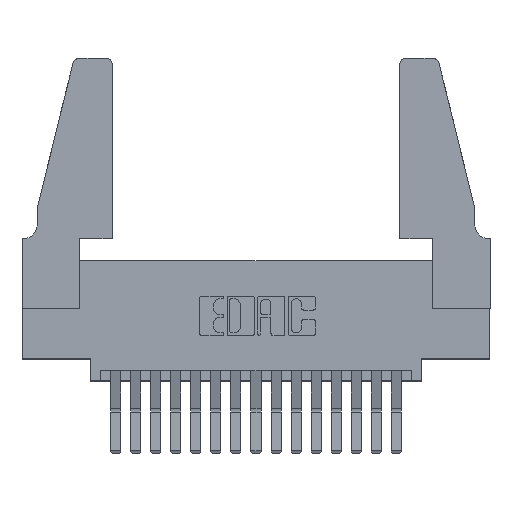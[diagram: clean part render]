
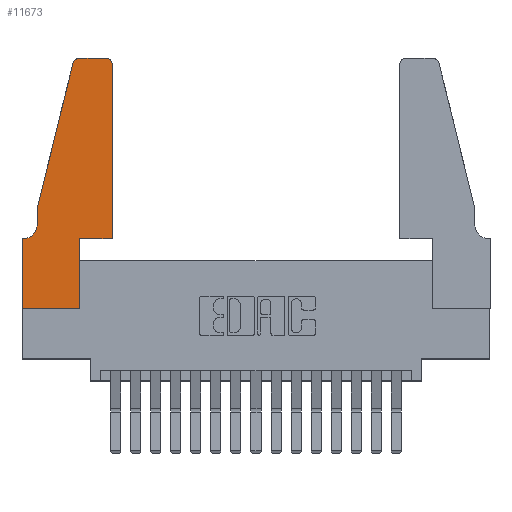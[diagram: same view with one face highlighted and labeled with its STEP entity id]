
A CAD part, top view. The second image highlights one B-rep face of the part: STEP entity #11673.
In plain terms, the highlighted planar face has unit normal (0, 0, 1).
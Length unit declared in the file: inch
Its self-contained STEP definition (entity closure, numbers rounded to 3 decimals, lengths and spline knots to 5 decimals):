
#372 = PLANE ( 'NONE',  #6034 ) ;
#391 = CARTESIAN_POINT ( 'NONE',  ( 0.2605, 1.25, 0.37 ) ) ;
#405 = VECTOR ( 'NONE', #438, 39.37008 ) ;
#438 = DIRECTION ( 'NONE',  ( 0., -1., 0. ) ) ;
#441 = CARTESIAN_POINT ( 'NONE',  ( 0.0755, 0.35, 0.37 ) ) ;
#473 = EDGE_CURVE ( 'NONE', #3197, #6181, #17310, .T. ) ;
#715 = CARTESIAN_POINT ( 'NONE',  ( 0., 0., 0.37 ) ) ;
#916 = VECTOR ( 'NONE', #14124, 39.37008 ) ;
#1012 = VECTOR ( 'NONE', #6200, 39.37008 ) ;
#1357 = DIRECTION ( 'NONE',  ( 1., 0., 0. ) ) ;
#1380 = CARTESIAN_POINT ( 'NONE',  ( 0., 0., 0.37 ) ) ;
#1688 = CARTESIAN_POINT ( 'NONE',  ( 0.4205, 1.25, 0.37 ) ) ;
#1715 = DIRECTION ( 'NONE',  ( 0., 0., 1. ) ) ;
#1775 = CARTESIAN_POINT ( 'NONE',  ( 0.4505, 0.35, 0.37 ) ) ;
#2473 = AXIS2_PLACEMENT_3D ( 'NONE', #11546, #9897, #15420 ) ;
#2487 = ORIENTED_EDGE ( 'NONE', *, *, #16562, .T. ) ;
#2564 = EDGE_CURVE ( 'NONE', #14074, #11543, #9876, .T. ) ;
#2922 = LINE ( 'NONE', #5318, #5719 ) ;
#3162 = DIRECTION ( 'NONE',  ( 0., 0., 1. ) ) ;
#3197 = VERTEX_POINT ( 'NONE', #17264 ) ;
#3398 = EDGE_CURVE ( 'NONE', #13388, #10427, #12030, .T. ) ;
#3519 = DIRECTION ( 'NONE',  ( 0., 1., 0. ) ) ;
#3649 = VERTEX_POINT ( 'NONE', #1775 ) ;
#4093 = ORIENTED_EDGE ( 'NONE', *, *, #11436, .T. ) ;
#4579 = DIRECTION ( 'NONE',  ( 0., 0., -1. ) ) ;
#4583 = CARTESIAN_POINT ( 'NONE',  ( 0.2865, 0., 0.37 ) ) ;
#4635 = VECTOR ( 'NONE', #5634, 39.37008 ) ;
#5318 = CARTESIAN_POINT ( 'NONE',  ( 0.4505, 0.35, 0.37 ) ) ;
#5634 = DIRECTION ( 'NONE',  ( -1., 0., 0. ) ) ;
#5673 = VERTEX_POINT ( 'NONE', #15279 ) ;
#5719 = VECTOR ( 'NONE', #12134, 39.37008 ) ;
#5816 = DIRECTION ( 'NONE',  ( 1., 0., 0. ) ) ;
#6004 = ORIENTED_EDGE ( 'NONE', *, *, #15431, .T. ) ;
#6034 = AXIS2_PLACEMENT_3D ( 'NONE', #14144, #3162, #8684 ) ;
#6181 = VERTEX_POINT ( 'NONE', #12402 ) ;
#6200 = DIRECTION ( 'NONE',  ( 1., 0., 0. ) ) ;
#6278 = CIRCLE ( 'NONE', #2473, 0.03 ) ;
#6533 = LINE ( 'NONE', #11529, #17296 ) ;
#6544 = FACE_OUTER_BOUND ( 'NONE', #16868, .T. ) ;
#6876 = CARTESIAN_POINT ( 'NONE',  ( 0.0755, 0.5, 0.37 ) ) ;
#7220 = DIRECTION ( 'NONE',  ( -1., 0., 0. ) ) ;
#8450 = ORIENTED_EDGE ( 'NONE', *, *, #473, .T. ) ;
#8670 = LINE ( 'NONE', #11311, #916 ) ;
#8684 = DIRECTION ( 'NONE',  ( 1., 0., 0. ) ) ;
#9327 = ORIENTED_EDGE ( 'NONE', *, *, #9500, .T. ) ;
#9500 = EDGE_CURVE ( 'NONE', #10845, #11806, #11365, .T. ) ;
#9577 = LINE ( 'NONE', #391, #4635 ) ;
#9876 = LINE ( 'NONE', #15399, #405 ) ;
#9897 = DIRECTION ( 'NONE',  ( 0., 0., 1. ) ) ;
#10202 = EDGE_CURVE ( 'NONE', #3649, #5673, #2922, .T. ) ;
#10216 = LINE ( 'NONE', #6876, #16232 ) ;
#10281 = ORIENTED_EDGE ( 'NONE', *, *, #10202, .T. ) ;
#10427 = VERTEX_POINT ( 'NONE', #4583 ) ;
#10845 = VERTEX_POINT ( 'NONE', #13632 ) ;
#10885 = EDGE_CURVE ( 'NONE', #12292, #3649, #16460, .T. ) ;
#11030 = DIRECTION ( 'NONE',  ( -0.239, -0.971, 0. ) ) ;
#11064 = AXIS2_PLACEMENT_3D ( 'NONE', #14232, #1715, #5816 ) ;
#11311 = CARTESIAN_POINT ( 'NONE',  ( 0., 0., 0.37 ) ) ;
#11365 = CIRCLE ( 'NONE', #11064, 0.03 ) ;
#11436 = EDGE_CURVE ( 'NONE', #11806, #14074, #10216, .T. ) ;
#11529 = CARTESIAN_POINT ( 'NONE',  ( 0.2865, 0.35, 0.37 ) ) ;
#11543 = VERTEX_POINT ( 'NONE', #13845 ) ;
#11546 = CARTESIAN_POINT ( 'NONE',  ( 0.4205, 1.22, 0.37 ) ) ;
#11548 = VERTEX_POINT ( 'NONE', #1688 ) ;
#11673 = ADVANCED_FACE ( 'NONE', ( #6544 ), #372, .T. ) ;
#11806 = VERTEX_POINT ( 'NONE', #11903 ) ;
#11883 = ORIENTED_EDGE ( 'NONE', *, *, #10885, .T. ) ;
#11903 = CARTESIAN_POINT ( 'NONE',  ( 0.25487, 1.22718, 0.37 ) ) ;
#12030 = LINE ( 'NONE', #715, #1012 ) ;
#12134 = DIRECTION ( 'NONE',  ( 0., 1., 0. ) ) ;
#12172 = ORIENTED_EDGE ( 'NONE', *, *, #17451, .T. ) ;
#12280 = CARTESIAN_POINT ( 'NONE',  ( 0.0755, 0.5, 0.37 ) ) ;
#12287 = EDGE_CURVE ( 'NONE', #6181, #13388, #8670, .T. ) ;
#12292 = VERTEX_POINT ( 'NONE', #16890 ) ;
#12402 = CARTESIAN_POINT ( 'NONE',  ( 0., 0.35, 0.37 ) ) ;
#12424 = AXIS2_PLACEMENT_3D ( 'NONE', #15568, #4579, #14301 ) ;
#12638 = CIRCLE ( 'NONE', #12424, 0.07 ) ;
#12857 = EDGE_CURVE ( 'NONE', #5673, #11548, #6278, .T. ) ;
#13234 = VECTOR ( 'NONE', #7220, 39.37008 ) ;
#13388 = VERTEX_POINT ( 'NONE', #1380 ) ;
#13632 = CARTESIAN_POINT ( 'NONE',  ( 0.284, 1.25, 0.37 ) ) ;
#13845 = CARTESIAN_POINT ( 'NONE',  ( 0.0755, 0.42, 0.37 ) ) ;
#14074 = VERTEX_POINT ( 'NONE', #12280 ) ;
#14124 = DIRECTION ( 'NONE',  ( 0., -1., 0. ) ) ;
#14144 = CARTESIAN_POINT ( 'NONE',  ( 0., 0.35, 0.37 ) ) ;
#14232 = CARTESIAN_POINT ( 'NONE',  ( 0.284, 1.22, 0.37 ) ) ;
#14301 = DIRECTION ( 'NONE',  ( -1., 0., 0. ) ) ;
#14818 = ORIENTED_EDGE ( 'NONE', *, *, #3398, .T. ) ;
#15078 = CARTESIAN_POINT ( 'NONE',  ( 0.4505, 0.35, 0.37 ) ) ;
#15279 = CARTESIAN_POINT ( 'NONE',  ( 0.4505, 1.22, 0.37 ) ) ;
#15399 = CARTESIAN_POINT ( 'NONE',  ( 0.0755, 0.5, 0.37 ) ) ;
#15420 = DIRECTION ( 'NONE',  ( 1., 0., 0. ) ) ;
#15431 = EDGE_CURVE ( 'NONE', #11543, #3197, #12638, .T. ) ;
#15568 = CARTESIAN_POINT ( 'NONE',  ( 0.0055, 0.42, 0.37 ) ) ;
#15616 = ORIENTED_EDGE ( 'NONE', *, *, #12857, .T. ) ;
#16232 = VECTOR ( 'NONE', #11030, 39.37008 ) ;
#16460 = LINE ( 'NONE', #15078, #17764 ) ;
#16562 = EDGE_CURVE ( 'NONE', #11548, #10845, #9577, .T. ) ;
#16682 = ORIENTED_EDGE ( 'NONE', *, *, #2564, .T. ) ;
#16868 = EDGE_LOOP ( 'NONE', ( #2487, #9327, #4093, #16682, #6004, #8450, #16946, #14818, #12172, #11883, #10281, #15616 ) ) ;
#16890 = CARTESIAN_POINT ( 'NONE',  ( 0.2865, 0.35, 0.37 ) ) ;
#16946 = ORIENTED_EDGE ( 'NONE', *, *, #12287, .T. ) ;
#17264 = CARTESIAN_POINT ( 'NONE',  ( 0.0055, 0.35, 0.37 ) ) ;
#17296 = VECTOR ( 'NONE', #3519, 39.37008 ) ;
#17310 = LINE ( 'NONE', #441, #13234 ) ;
#17451 = EDGE_CURVE ( 'NONE', #10427, #12292, #6533, .T. ) ;
#17764 = VECTOR ( 'NONE', #1357, 39.37008 ) ;
